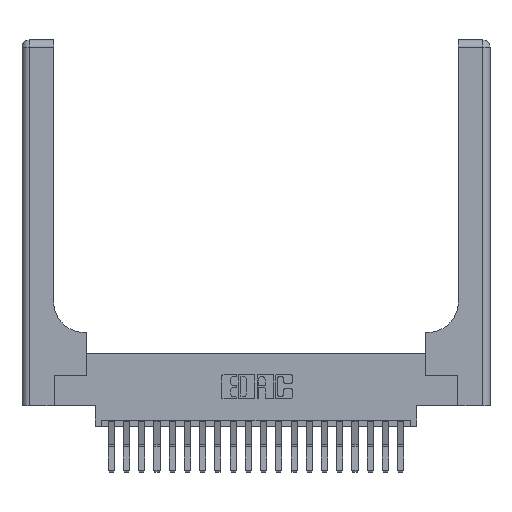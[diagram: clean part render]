
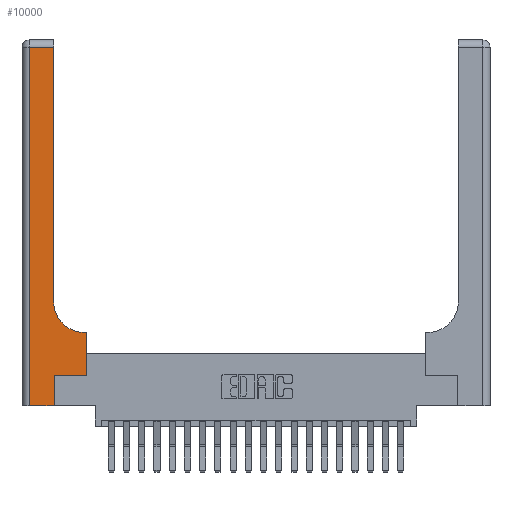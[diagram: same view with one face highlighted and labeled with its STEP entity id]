
A CAD part, top view. The second image highlights one B-rep face of the part: STEP entity #10000.
In plain terms, the highlighted planar face has unit normal (0, 0, 1).
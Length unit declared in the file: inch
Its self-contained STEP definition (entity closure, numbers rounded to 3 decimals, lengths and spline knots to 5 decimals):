
#497 = PLANE ( 'NONE',  #3554 ) ;
#592 = CARTESIAN_POINT ( 'NONE',  ( 0.06, 0., 0.37 ) ) ;
#779 = DIRECTION ( 'NONE',  ( -1., 0., 0. ) ) ;
#1370 = DIRECTION ( 'NONE',  ( 0., 1., 0. ) ) ;
#1445 = CARTESIAN_POINT ( 'NONE',  ( 0.26, 2.94, 0.37 ) ) ;
#1625 = EDGE_CURVE ( 'NONE', #15868, #20393, #3872, .T. ) ;
#2058 = CARTESIAN_POINT ( 'NONE',  ( 0.528, 0.25, 0.37 ) ) ;
#2488 = DIRECTION ( 'NONE',  ( -1., 0., 0. ) ) ;
#2751 = CARTESIAN_POINT ( 'NONE',  ( 0.528, 0.25, 0.37 ) ) ;
#3431 = VERTEX_POINT ( 'NONE', #4318 ) ;
#3554 = AXIS2_PLACEMENT_3D ( 'NONE', #5355, #17632, #2488 ) ;
#3761 = CARTESIAN_POINT ( 'NONE',  ( 0.06, 3., 0.37 ) ) ;
#3872 = LINE ( 'NONE', #3761, #15554 ) ;
#4318 = CARTESIAN_POINT ( 'NONE',  ( 0.265, 0.25, 0.37 ) ) ;
#4337 = CARTESIAN_POINT ( 'NONE',  ( 0., 0., 0.37 ) ) ;
#4994 = ORIENTED_EDGE ( 'NONE', *, *, #18327, .T. ) ;
#5221 = VERTEX_POINT ( 'NONE', #2751 ) ;
#5355 = CARTESIAN_POINT ( 'NONE',  ( 0., 3., 0.37 ) ) ;
#5503 = ORIENTED_EDGE ( 'NONE', *, *, #10093, .T. ) ;
#5542 = VECTOR ( 'NONE', #11465, 39.37008 ) ;
#5586 = VECTOR ( 'NONE', #8796, 39.37008 ) ;
#6232 = CARTESIAN_POINT ( 'NONE',  ( 0.26, 3., 0.37 ) ) ;
#7145 = VERTEX_POINT ( 'NONE', #10921 ) ;
#7299 = VECTOR ( 'NONE', #779, 39.37008 ) ;
#8286 = CARTESIAN_POINT ( 'NONE',  ( 0.06, 2.94, 0.37 ) ) ;
#8376 = VECTOR ( 'NONE', #9207, 39.37008 ) ;
#8519 = ORIENTED_EDGE ( 'NONE', *, *, #20472, .T. ) ;
#8796 = DIRECTION ( 'NONE',  ( 0., 1., 0. ) ) ;
#8824 = VERTEX_POINT ( 'NONE', #12443 ) ;
#9207 = DIRECTION ( 'NONE',  ( 1., 0., 0. ) ) ;
#9416 = CARTESIAN_POINT ( 'NONE',  ( 0.26, 0.6, 0.37 ) ) ;
#9531 = VERTEX_POINT ( 'NONE', #10813 ) ;
#10000 = ADVANCED_FACE ( 'NONE', ( #13874 ), #497, .F. ) ;
#10093 = EDGE_CURVE ( 'NONE', #7145, #3431, #10903, .T. ) ;
#10622 = DIRECTION ( 'NONE',  ( 0., -1., 0. ) ) ;
#10652 = LINE ( 'NONE', #9416, #16692 ) ;
#10813 = CARTESIAN_POINT ( 'NONE',  ( 0.51, 0.6, 0.37 ) ) ;
#10903 = LINE ( 'NONE', #20730, #18039 ) ;
#10914 = ORIENTED_EDGE ( 'NONE', *, *, #12771, .T. ) ;
#10921 = CARTESIAN_POINT ( 'NONE',  ( 0.265, 0., 0.37 ) ) ;
#11035 = ORIENTED_EDGE ( 'NONE', *, *, #21593, .T. ) ;
#11060 = ORIENTED_EDGE ( 'NONE', *, *, #13407, .T. ) ;
#11465 = DIRECTION ( 'NONE',  ( 1., 0., 0. ) ) ;
#11763 = CARTESIAN_POINT ( 'NONE',  ( 0.51, 0.85, 0.37 ) ) ;
#12317 = DIRECTION ( 'NONE',  ( -1., 0., 0. ) ) ;
#12443 = CARTESIAN_POINT ( 'NONE',  ( 0.26, 0.85, 0.37 ) ) ;
#12451 = DIRECTION ( 'NONE',  ( 0., 1., 0. ) ) ;
#12616 = LINE ( 'NONE', #12824, #7299 ) ;
#12644 = LINE ( 'NONE', #4337, #8376 ) ;
#12771 = EDGE_CURVE ( 'NONE', #3431, #5221, #21629, .T. ) ;
#12824 = CARTESIAN_POINT ( 'NONE',  ( 0., 2.94, 0.37 ) ) ;
#13009 = CARTESIAN_POINT ( 'NONE',  ( 0.265, 0.25, 0.37 ) ) ;
#13095 = EDGE_CURVE ( 'NONE', #8824, #15883, #16521, .T. ) ;
#13214 = VERTEX_POINT ( 'NONE', #18829 ) ;
#13231 = EDGE_LOOP ( 'NONE', ( #13949, #13983, #18192, #8519, #5503, #10914, #11035, #11060, #4994 ) ) ;
#13407 = EDGE_CURVE ( 'NONE', #13214, #9531, #10652, .T. ) ;
#13874 = FACE_OUTER_BOUND ( 'NONE', #13231, .T. ) ;
#13949 = ORIENTED_EDGE ( 'NONE', *, *, #13095, .T. ) ;
#13983 = ORIENTED_EDGE ( 'NONE', *, *, #19557, .T. ) ;
#15554 = VECTOR ( 'NONE', #10622, 39.37008 ) ;
#15868 = VERTEX_POINT ( 'NONE', #8286 ) ;
#15883 = VERTEX_POINT ( 'NONE', #1445 ) ;
#16521 = LINE ( 'NONE', #6232, #16801 ) ;
#16692 = VECTOR ( 'NONE', #12317, 39.37008 ) ;
#16801 = VECTOR ( 'NONE', #1370, 39.37008 ) ;
#17149 = CIRCLE ( 'NONE', #17511, 0.25 ) ;
#17511 = AXIS2_PLACEMENT_3D ( 'NONE', #11763, #21603, #19953 ) ;
#17632 = DIRECTION ( 'NONE',  ( 0., 0., -1. ) ) ;
#18039 = VECTOR ( 'NONE', #12451, 39.37008 ) ;
#18192 = ORIENTED_EDGE ( 'NONE', *, *, #1625, .T. ) ;
#18327 = EDGE_CURVE ( 'NONE', #9531, #8824, #17149, .T. ) ;
#18829 = CARTESIAN_POINT ( 'NONE',  ( 0.528, 0.6, 0.37 ) ) ;
#19557 = EDGE_CURVE ( 'NONE', #15883, #15868, #12616, .T. ) ;
#19953 = DIRECTION ( 'NONE',  ( 1., 0., 0. ) ) ;
#20393 = VERTEX_POINT ( 'NONE', #592 ) ;
#20416 = LINE ( 'NONE', #2058, #5586 ) ;
#20472 = EDGE_CURVE ( 'NONE', #20393, #7145, #12644, .T. ) ;
#20730 = CARTESIAN_POINT ( 'NONE',  ( 0.265, 0., 0.37 ) ) ;
#21593 = EDGE_CURVE ( 'NONE', #5221, #13214, #20416, .T. ) ;
#21603 = DIRECTION ( 'NONE',  ( 0., 0., -1. ) ) ;
#21629 = LINE ( 'NONE', #13009, #5542 ) ;
